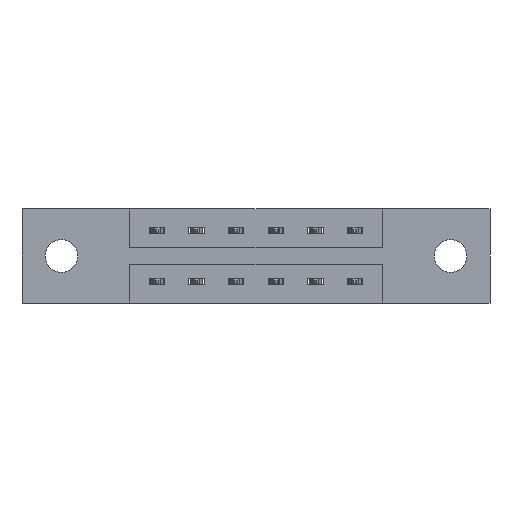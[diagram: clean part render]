
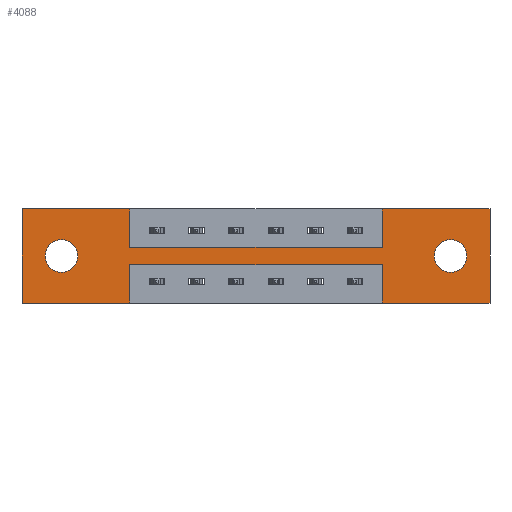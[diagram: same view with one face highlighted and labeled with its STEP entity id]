
A CAD part, front view. The second image highlights one B-rep face of the part: STEP entity #4088.
In plain terms, the highlighted planar face has unit normal (0, -1, 0).
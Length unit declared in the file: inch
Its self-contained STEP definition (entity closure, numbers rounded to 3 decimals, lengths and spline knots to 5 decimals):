
#6 = LINE ( 'NONE', #5029, #1735 ) ;
#55 = CARTESIAN_POINT ( 'NONE',  ( 1.687, 0., -0.121 ) ) ;
#170 = CARTESIAN_POINT ( 'NONE',  ( 0., 0., -0.37 ) ) ;
#243 = DIRECTION ( 'NONE',  ( 0., 0., 1. ) ) ;
#287 = CARTESIAN_POINT ( 'NONE',  ( 0.425, 0., -0.37 ) ) ;
#369 = DIRECTION ( 'NONE',  ( 0., 0., 1. ) ) ;
#411 = CARTESIAN_POINT ( 'NONE',  ( 0., 0., 0. ) ) ;
#418 = CARTESIAN_POINT ( 'NONE',  ( 0.425, 0., -0.22 ) ) ;
#531 = EDGE_CURVE ( 'NONE', #4362, #3893, #6, .T. ) ;
#545 = EDGE_CURVE ( 'NONE', #1275, #3315, #3731, .T. ) ;
#625 = AXIS2_PLACEMENT_3D ( 'NONE', #680, #8829, #1521 ) ;
#680 = CARTESIAN_POINT ( 'NONE',  ( 0.155, 0., -0.185 ) ) ;
#683 = CARTESIAN_POINT ( 'NONE',  ( 0.425, 0., 0. ) ) ;
#817 = VECTOR ( 'NONE', #6407, 39.37008 ) ;
#862 = CARTESIAN_POINT ( 'NONE',  ( 1.417, 0., 0. ) ) ;
#998 = PLANE ( 'NONE',  #8356 ) ;
#1058 = VECTOR ( 'NONE', #3037, 39.37008 ) ;
#1210 = VECTOR ( 'NONE', #369, 39.37008 ) ;
#1271 = VERTEX_POINT ( 'NONE', #418 ) ;
#1275 = VERTEX_POINT ( 'NONE', #8220 ) ;
#1483 = VECTOR ( 'NONE', #8223, 39.37008 ) ;
#1521 = DIRECTION ( 'NONE',  ( 0., 0., 1. ) ) ;
#1557 = VERTEX_POINT ( 'NONE', #8616 ) ;
#1704 = VECTOR ( 'NONE', #9075, 39.37008 ) ;
#1735 = VECTOR ( 'NONE', #5615, 39.37008 ) ;
#1883 = VECTOR ( 'NONE', #3420, 39.37008 ) ;
#1963 = CARTESIAN_POINT ( 'NONE',  ( 1.687, 0., -0.185 ) ) ;
#2027 = VECTOR ( 'NONE', #6564, 39.37008 ) ;
#2048 = EDGE_CURVE ( 'NONE', #9286, #6746, #7580, .T. ) ;
#2115 = DIRECTION ( 'NONE',  ( 1., 0., 0. ) ) ;
#2168 = VECTOR ( 'NONE', #8165, 39.37008 ) ;
#2243 = CARTESIAN_POINT ( 'NONE',  ( 0.425, 0., -0.22 ) ) ;
#2454 = VERTEX_POINT ( 'NONE', #8184 ) ;
#2458 = EDGE_CURVE ( 'NONE', #6974, #1557, #3696, .T. ) ;
#2533 = FACE_BOUND ( 'NONE', #6500, .T. ) ;
#2598 = CARTESIAN_POINT ( 'NONE',  ( 1.687, 0., -0.249 ) ) ;
#2666 = CARTESIAN_POINT ( 'NONE',  ( 1.842, 0., 0. ) ) ;
#2680 = EDGE_CURVE ( 'NONE', #6746, #4362, #4051, .T. ) ;
#2725 = EDGE_CURVE ( 'NONE', #3860, #8533, #7464, .T. ) ;
#2817 = DIRECTION ( 'NONE',  ( 0., 1., 0. ) ) ;
#3037 = DIRECTION ( 'NONE',  ( 1., 0., 0. ) ) ;
#3092 = CARTESIAN_POINT ( 'NONE',  ( 0.425, 0., -0.15 ) ) ;
#3165 = LINE ( 'NONE', #3327, #1210 ) ;
#3203 = LINE ( 'NONE', #8543, #1483 ) ;
#3229 = EDGE_CURVE ( 'NONE', #8504, #1271, #4902, .T. ) ;
#3305 = CARTESIAN_POINT ( 'NONE',  ( 1.417, 0., -0.22 ) ) ;
#3315 = VERTEX_POINT ( 'NONE', #4274 ) ;
#3327 = CARTESIAN_POINT ( 'NONE',  ( 1.417, 0., -0.37 ) ) ;
#3420 = DIRECTION ( 'NONE',  ( 0., 0., -1. ) ) ;
#3696 = LINE ( 'NONE', #3800, #1704 ) ;
#3731 = CIRCLE ( 'NONE', #625, 0.064 ) ;
#3784 = DIRECTION ( 'NONE',  ( -1., 0., 0. ) ) ;
#3800 = CARTESIAN_POINT ( 'NONE',  ( 0., 0., -0.37 ) ) ;
#3844 = ORIENTED_EDGE ( 'NONE', *, *, #2725, .T. ) ;
#3860 = VERTEX_POINT ( 'NONE', #55 ) ;
#3893 = VERTEX_POINT ( 'NONE', #683 ) ;
#3930 = ORIENTED_EDGE ( 'NONE', *, *, #9271, .T. ) ;
#3959 = ORIENTED_EDGE ( 'NONE', *, *, #545, .T. ) ;
#3987 = ORIENTED_EDGE ( 'NONE', *, *, #7906, .T. ) ;
#4026 = CARTESIAN_POINT ( 'NONE',  ( 1.687, 0., -0.185 ) ) ;
#4051 = LINE ( 'NONE', #411, #2027 ) ;
#4058 = ORIENTED_EDGE ( 'NONE', *, *, #4293, .F. ) ;
#4069 = ORIENTED_EDGE ( 'NONE', *, *, #3229, .F. ) ;
#4086 = ORIENTED_EDGE ( 'NONE', *, *, #2680, .F. ) ;
#4088 = ADVANCED_FACE ( 'NONE', ( #2533, #6063, #7917 ), #998, .T. ) ;
#4109 = ORIENTED_EDGE ( 'NONE', *, *, #7217, .F. ) ;
#4159 = ORIENTED_EDGE ( 'NONE', *, *, #9074, .F. ) ;
#4176 = CARTESIAN_POINT ( 'NONE',  ( 1.417, 0., -0.15 ) ) ;
#4189 = ORIENTED_EDGE ( 'NONE', *, *, #8587, .F. ) ;
#4200 = ORIENTED_EDGE ( 'NONE', *, *, #8408, .F. ) ;
#4221 = ORIENTED_EDGE ( 'NONE', *, *, #4820, .F. ) ;
#4224 = ORIENTED_EDGE ( 'NONE', *, *, #8191, .F. ) ;
#4245 = ORIENTED_EDGE ( 'NONE', *, *, #2458, .F. ) ;
#4264 = VECTOR ( 'NONE', #2115, 39.37008 ) ;
#4274 = CARTESIAN_POINT ( 'NONE',  ( 0.155, 0., -0.249 ) ) ;
#4275 = CIRCLE ( 'NONE', #7511, 0.064 ) ;
#4293 = EDGE_CURVE ( 'NONE', #1271, #9286, #3203, .T. ) ;
#4362 = VERTEX_POINT ( 'NONE', #7462 ) ;
#4766 = DIRECTION ( 'NONE',  ( 0., 1., 0. ) ) ;
#4817 = DIRECTION ( 'NONE',  ( 0., 0., 1. ) ) ;
#4819 = DIRECTION ( 'NONE',  ( 0., 0., -1. ) ) ;
#4820 = EDGE_CURVE ( 'NONE', #8586, #2454, #6383, .T. ) ;
#4902 = LINE ( 'NONE', #2243, #6799 ) ;
#4997 = CARTESIAN_POINT ( 'NONE',  ( 1.842, 0., 0. ) ) ;
#5029 = CARTESIAN_POINT ( 'NONE',  ( 0., 0., 0. ) ) ;
#5197 = ORIENTED_EDGE ( 'NONE', *, *, #2048, .F. ) ;
#5572 = DIRECTION ( 'NONE',  ( 0., 0., -1. ) ) ;
#5615 = DIRECTION ( 'NONE',  ( 1., 0., 0. ) ) ;
#5654 = CIRCLE ( 'NONE', #7796, 0.064 ) ;
#5918 = CARTESIAN_POINT ( 'NONE',  ( 0., 0., -0.37 ) ) ;
#6063 = FACE_BOUND ( 'NONE', #6639, .T. ) ;
#6078 = CARTESIAN_POINT ( 'NONE',  ( 1.842, 0., -0.37 ) ) ;
#6085 = CARTESIAN_POINT ( 'NONE',  ( 0.425, 0., -0.15 ) ) ;
#6217 = LINE ( 'NONE', #8630, #4264 ) ;
#6305 = CARTESIAN_POINT ( 'NONE',  ( 0., 0., -0.37 ) ) ;
#6333 = DIRECTION ( 'NONE',  ( 0., -1., 0. ) ) ;
#6383 = LINE ( 'NONE', #862, #8216 ) ;
#6407 = DIRECTION ( 'NONE',  ( 0., 0., -1. ) ) ;
#6500 = EDGE_LOOP ( 'NONE', ( #3844, #3930 ) ) ;
#6564 = DIRECTION ( 'NONE',  ( 0., 0., 1. ) ) ;
#6639 = EDGE_LOOP ( 'NONE', ( #3959, #3987 ) ) ;
#6746 = VERTEX_POINT ( 'NONE', #5918 ) ;
#6799 = VECTOR ( 'NONE', #3784, 39.37008 ) ;
#6974 = VERTEX_POINT ( 'NONE', #6078 ) ;
#6990 = LINE ( 'NONE', #6085, #1058 ) ;
#7039 = VERTEX_POINT ( 'NONE', #3092 ) ;
#7217 = EDGE_CURVE ( 'NONE', #1557, #8504, #3165, .T. ) ;
#7305 = VERTEX_POINT ( 'NONE', #4997 ) ;
#7454 = EDGE_LOOP ( 'NONE', ( #4058, #4069, #4109, #4245, #4224, #4200, #4221, #4159, #4189, #8353, #4086, #5197 ) ) ;
#7462 = CARTESIAN_POINT ( 'NONE',  ( 0., 0., 0. ) ) ;
#7464 = CIRCLE ( 'NONE', #7640, 0.064 ) ;
#7467 = DIRECTION ( 'NONE',  ( 0., 0., -1. ) ) ;
#7511 = AXIS2_PLACEMENT_3D ( 'NONE', #8956, #4766, #243 ) ;
#7580 = LINE ( 'NONE', #170, #2168 ) ;
#7640 = AXIS2_PLACEMENT_3D ( 'NONE', #1963, #2817, #5572 ) ;
#7748 = LINE ( 'NONE', #2666, #1883 ) ;
#7796 = AXIS2_PLACEMENT_3D ( 'NONE', #4026, #9000, #4819 ) ;
#7906 = EDGE_CURVE ( 'NONE', #3315, #1275, #4275, .T. ) ;
#7917 = FACE_OUTER_BOUND ( 'NONE', #7454, .T. ) ;
#8165 = DIRECTION ( 'NONE',  ( -1., 0., 0. ) ) ;
#8184 = CARTESIAN_POINT ( 'NONE',  ( 1.417, 0., 0. ) ) ;
#8191 = EDGE_CURVE ( 'NONE', #7305, #6974, #7748, .T. ) ;
#8216 = VECTOR ( 'NONE', #4817, 39.37008 ) ;
#8220 = CARTESIAN_POINT ( 'NONE',  ( 0.155, 0., -0.121 ) ) ;
#8223 = DIRECTION ( 'NONE',  ( 0., 0., -1. ) ) ;
#8353 = ORIENTED_EDGE ( 'NONE', *, *, #531, .F. ) ;
#8356 = AXIS2_PLACEMENT_3D ( 'NONE', #6305, #6333, #7467 ) ;
#8408 = EDGE_CURVE ( 'NONE', #2454, #7305, #6217, .T. ) ;
#8504 = VERTEX_POINT ( 'NONE', #3305 ) ;
#8533 = VERTEX_POINT ( 'NONE', #2598 ) ;
#8543 = CARTESIAN_POINT ( 'NONE',  ( 0.425, 0., -0.37 ) ) ;
#8586 = VERTEX_POINT ( 'NONE', #4176 ) ;
#8587 = EDGE_CURVE ( 'NONE', #3893, #7039, #8596, .T. ) ;
#8596 = LINE ( 'NONE', #9106, #817 ) ;
#8616 = CARTESIAN_POINT ( 'NONE',  ( 1.417, 0., -0.37 ) ) ;
#8630 = CARTESIAN_POINT ( 'NONE',  ( 0., 0., 0. ) ) ;
#8829 = DIRECTION ( 'NONE',  ( 0., 1., 0. ) ) ;
#8956 = CARTESIAN_POINT ( 'NONE',  ( 0.155, 0., -0.185 ) ) ;
#9000 = DIRECTION ( 'NONE',  ( 0., 1., 0. ) ) ;
#9074 = EDGE_CURVE ( 'NONE', #7039, #8586, #6990, .T. ) ;
#9075 = DIRECTION ( 'NONE',  ( -1., 0., 0. ) ) ;
#9106 = CARTESIAN_POINT ( 'NONE',  ( 0.425, 0., 0. ) ) ;
#9271 = EDGE_CURVE ( 'NONE', #8533, #3860, #5654, .T. ) ;
#9286 = VERTEX_POINT ( 'NONE', #287 ) ;
